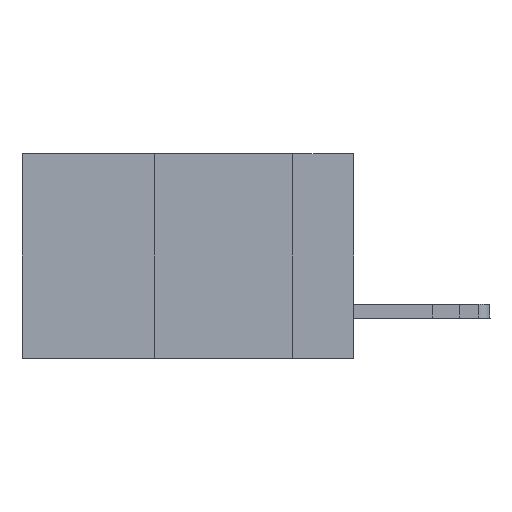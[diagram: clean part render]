
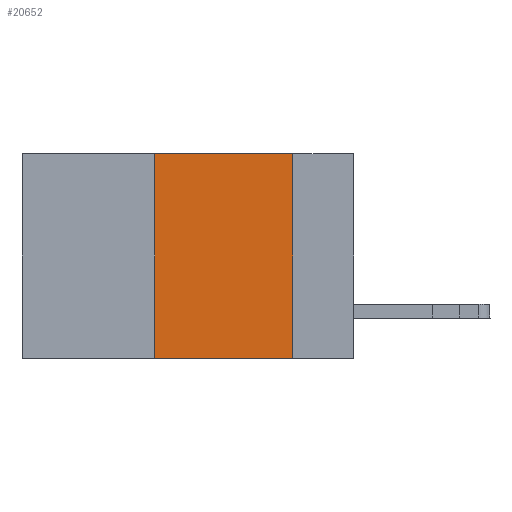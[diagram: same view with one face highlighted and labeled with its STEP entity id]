
A CAD part, left-side view. The second image highlights one B-rep face of the part: STEP entity #20652.
In plain terms, the highlighted planar face has unit normal (-1, 0, 0).
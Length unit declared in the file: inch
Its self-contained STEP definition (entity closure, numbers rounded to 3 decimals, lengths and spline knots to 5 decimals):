
#849 = VERTEX_POINT ( 'NONE', #21485 ) ;
#1270 = DIRECTION ( 'NONE',  ( 0., 0., 1. ) ) ;
#4189 = FACE_OUTER_BOUND ( 'NONE', #15301, .T. ) ;
#4207 = VERTEX_POINT ( 'NONE', #21828 ) ;
#4954 = VERTEX_POINT ( 'NONE', #10584 ) ;
#4994 = CARTESIAN_POINT ( 'NONE',  ( 0., 0.6, 0. ) ) ;
#5295 = EDGE_CURVE ( 'NONE', #4954, #14969, #14139, .T. ) ;
#6590 = ORIENTED_EDGE ( 'NONE', *, *, #5295, .F. ) ;
#7845 = EDGE_CURVE ( 'NONE', #4207, #14969, #12915, .T. ) ;
#8060 = ORIENTED_EDGE ( 'NONE', *, *, #14235, .F. ) ;
#8133 = VECTOR ( 'NONE', #28472, 39.37008 ) ;
#8404 = VECTOR ( 'NONE', #1270, 39.37008 ) ;
#9611 = AXIS2_PLACEMENT_3D ( 'NONE', #4994, #11932, #27365 ) ;
#9747 = CARTESIAN_POINT ( 'NONE',  ( 0., 0.6, 0. ) ) ;
#10584 = CARTESIAN_POINT ( 'NONE',  ( 0., 0.11, 0. ) ) ;
#11932 = DIRECTION ( 'NONE',  ( 1., 0., 0. ) ) ;
#12224 = VECTOR ( 'NONE', #15529, 39.37008 ) ;
#12915 = LINE ( 'NONE', #13288, #12224 ) ;
#13288 = CARTESIAN_POINT ( 'NONE',  ( 0., 0.6, -0.37 ) ) ;
#14139 = LINE ( 'NONE', #28375, #8133 ) ;
#14235 = EDGE_CURVE ( 'NONE', #849, #4954, #26275, .T. ) ;
#14969 = VERTEX_POINT ( 'NONE', #25531 ) ;
#15068 = CARTESIAN_POINT ( 'NONE',  ( 0., 0.36, 0. ) ) ;
#15301 = EDGE_LOOP ( 'NONE', ( #6590, #8060, #25061, #26096 ) ) ;
#15529 = DIRECTION ( 'NONE',  ( 0., -1., 0. ) ) ;
#20245 = LINE ( 'NONE', #15068, #8404 ) ;
#20652 = ADVANCED_FACE ( 'NONE', ( #4189 ), #27279, .F. ) ;
#21090 = VECTOR ( 'NONE', #25282, 39.37008 ) ;
#21485 = CARTESIAN_POINT ( 'NONE',  ( 0., 0.36, 0. ) ) ;
#21828 = CARTESIAN_POINT ( 'NONE',  ( 0., 0.36, -0.37 ) ) ;
#25061 = ORIENTED_EDGE ( 'NONE', *, *, #27724, .F. ) ;
#25282 = DIRECTION ( 'NONE',  ( 0., -1., 0. ) ) ;
#25531 = CARTESIAN_POINT ( 'NONE',  ( 0., 0.11, -0.37 ) ) ;
#26096 = ORIENTED_EDGE ( 'NONE', *, *, #7845, .T. ) ;
#26275 = LINE ( 'NONE', #9747, #21090 ) ;
#27279 = PLANE ( 'NONE',  #9611 ) ;
#27365 = DIRECTION ( 'NONE',  ( 0., 0., -1. ) ) ;
#27724 = EDGE_CURVE ( 'NONE', #4207, #849, #20245, .T. ) ;
#28375 = CARTESIAN_POINT ( 'NONE',  ( 0., 0.11, 0. ) ) ;
#28472 = DIRECTION ( 'NONE',  ( 0., 0., -1. ) ) ;
